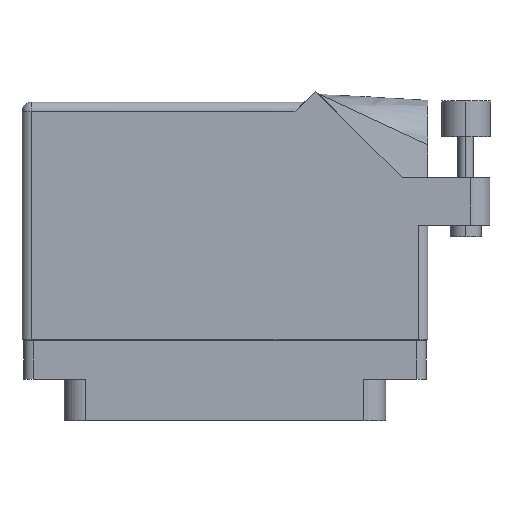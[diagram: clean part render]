
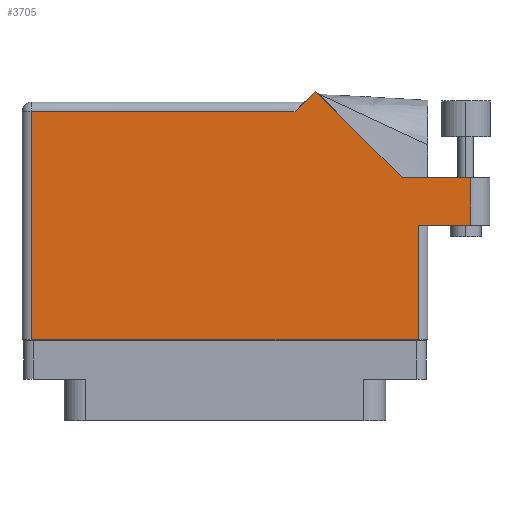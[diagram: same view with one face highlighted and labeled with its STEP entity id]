
A CAD part, front view. The second image highlights one B-rep face of the part: STEP entity #3705.
In plain terms, the highlighted face is planar.
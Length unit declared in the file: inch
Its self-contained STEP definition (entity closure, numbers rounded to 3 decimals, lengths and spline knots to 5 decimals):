
#301 = VERTEX_POINT ( 'NONE', #27446 ) ;
#938 = DIRECTION ( 'NONE',  ( 0., 1., 0. ) ) ;
#2329 = CARTESIAN_POINT ( 'NONE',  ( 1.244, 0.637, 0.455 ) ) ;
#2551 = ORIENTED_EDGE ( 'NONE', *, *, #46005, .T. ) ;
#3321 = EDGE_CURVE ( 'NONE', #7076, #5929, #33077, .T. ) ;
#3705 = ADVANCED_FACE ( 'NONE', ( #27826 ), #24356, .F. ) ;
#5131 = LINE ( 'NONE', #43101, #43248 ) ;
#5236 = VECTOR ( 'NONE', #36275, 39.37008 ) ;
#5355 = ORIENTED_EDGE ( 'NONE', *, *, #12656, .T. ) ;
#5929 = VERTEX_POINT ( 'NONE', #25314 ) ;
#6351 = CARTESIAN_POINT ( 'NONE',  ( -1.306, 1.368, 0.455 ) ) ;
#6507 = DIRECTION ( 'NONE',  ( -1., 0., 0. ) ) ;
#6863 = DIRECTION ( 'NONE',  ( 1., 0., 0. ) ) ;
#6996 = DIRECTION ( 'NONE',  ( -1., 0., 0. ) ) ;
#7076 = VERTEX_POINT ( 'NONE', #7774 ) ;
#7752 = ORIENTED_EDGE ( 'NONE', *, *, #3321, .T. ) ;
#7774 = CARTESIAN_POINT ( 'NONE',  ( 1.244, 0.637, 0.455 ) ) ;
#8053 = CARTESIAN_POINT ( 'NONE',  ( 1.581, 0.944, 0.455 ) ) ;
#8948 = ORIENTED_EDGE ( 'NONE', *, *, #35628, .T. ) ;
#9172 = LINE ( 'NONE', #17972, #5236 ) ;
#11012 = CARTESIAN_POINT ( 'NONE',  ( 1.706, 0.944, 0.455 ) ) ;
#11479 = CARTESIAN_POINT ( 'NONE',  ( -1.244, 1.368, 0.455 ) ) ;
#12656 = EDGE_CURVE ( 'NONE', #14174, #14390, #27420, .T. ) ;
#13415 = EDGE_CURVE ( 'NONE', #14390, #25380, #39496, .T. ) ;
#13550 = AXIS2_PLACEMENT_3D ( 'NONE', #39416, #39259, #17106 ) ;
#13597 = VECTOR ( 'NONE', #13934, 39.37008 ) ;
#13934 = DIRECTION ( 'NONE',  ( -0.707, -0.707, 0. ) ) ;
#14174 = VERTEX_POINT ( 'NONE', #34698 ) ;
#14390 = VERTEX_POINT ( 'NONE', #28225 ) ;
#15203 = VECTOR ( 'NONE', #6507, 39.37008 ) ;
#17106 = DIRECTION ( 'NONE',  ( -1., 0., 0. ) ) ;
#17291 = LINE ( 'NONE', #37040, #42700 ) ;
#17882 = CARTESIAN_POINT ( 'NONE',  ( 1.14042, 0.944, 0.455 ) ) ;
#17972 = CARTESIAN_POINT ( 'NONE',  ( -1.244, -0.1, 0.455 ) ) ;
#18172 = VECTOR ( 'NONE', #31569, 39.37008 ) ;
#21081 = ORIENTED_EDGE ( 'NONE', *, *, #21237, .T. ) ;
#21237 = EDGE_CURVE ( 'NONE', #5929, #301, #41864, .T. ) ;
#23212 = VECTOR ( 'NONE', #43210, 39.37008 ) ;
#24356 = PLANE ( 'NONE',  #13550 ) ;
#25314 = CARTESIAN_POINT ( 'NONE',  ( 1.581, 0.637, 0.455 ) ) ;
#25380 = VERTEX_POINT ( 'NONE', #11479 ) ;
#25832 = EDGE_CURVE ( 'NONE', #38977, #7076, #41295, .T. ) ;
#27420 = LINE ( 'NONE', #35621, #13597 ) ;
#27446 = CARTESIAN_POINT ( 'NONE',  ( 1.581, 0.944, 0.455 ) ) ;
#27452 = ORIENTED_EDGE ( 'NONE', *, *, #25832, .T. ) ;
#27723 = CARTESIAN_POINT ( 'NONE',  ( 1.306, 0.637, 0.455 ) ) ;
#27826 = FACE_OUTER_BOUND ( 'NONE', #33611, .T. ) ;
#27966 = ORIENTED_EDGE ( 'NONE', *, *, #13415, .T. ) ;
#28225 = CARTESIAN_POINT ( 'NONE',  ( 0.451, 1.368, 0.455 ) ) ;
#28959 = ORIENTED_EDGE ( 'NONE', *, *, #35350, .T. ) ;
#30722 = VERTEX_POINT ( 'NONE', #36775 ) ;
#31569 = DIRECTION ( 'NONE',  ( 0., 1., 0. ) ) ;
#33077 = LINE ( 'NONE', #27723, #23212 ) ;
#33611 = EDGE_LOOP ( 'NONE', ( #7752, #21081, #2551, #8948, #5355, #27966, #39961, #28959, #27452 ) ) ;
#34698 = CARTESIAN_POINT ( 'NONE',  ( 0.58371, 1.50071, 0.455 ) ) ;
#35350 = EDGE_CURVE ( 'NONE', #30722, #38977, #17291, .T. ) ;
#35621 = CARTESIAN_POINT ( 'NONE',  ( 0.513, 1.43, 0.455 ) ) ;
#35628 = EDGE_CURVE ( 'NONE', #43374, #14174, #5131, .T. ) ;
#36275 = DIRECTION ( 'NONE',  ( 0., -1., 0. ) ) ;
#36775 = CARTESIAN_POINT ( 'NONE',  ( -1.244, -0.1, 0.455 ) ) ;
#37040 = CARTESIAN_POINT ( 'NONE',  ( -1.306, -0.1, 0.455 ) ) ;
#37290 = VECTOR ( 'NONE', #938, 39.37008 ) ;
#37399 = LINE ( 'NONE', #11012, #40250 ) ;
#38977 = VERTEX_POINT ( 'NONE', #46409 ) ;
#39259 = DIRECTION ( 'NONE',  ( 0., 0., -1. ) ) ;
#39416 = CARTESIAN_POINT ( 'NONE',  ( -1.306, 1.43, 0.455 ) ) ;
#39496 = LINE ( 'NONE', #6351, #15203 ) ;
#39961 = ORIENTED_EDGE ( 'NONE', *, *, #43880, .T. ) ;
#40250 = VECTOR ( 'NONE', #6996, 39.37008 ) ;
#41123 = DIRECTION ( 'NONE',  ( -0.707, 0.707, 0. ) ) ;
#41295 = LINE ( 'NONE', #2329, #18172 ) ;
#41864 = LINE ( 'NONE', #8053, #37290 ) ;
#42700 = VECTOR ( 'NONE', #6863, 39.37008 ) ;
#43101 = CARTESIAN_POINT ( 'NONE',  ( 1.14042, 0.944, 0.455 ) ) ;
#43210 = DIRECTION ( 'NONE',  ( 1., 0., 0. ) ) ;
#43248 = VECTOR ( 'NONE', #41123, 39.37008 ) ;
#43374 = VERTEX_POINT ( 'NONE', #17882 ) ;
#43880 = EDGE_CURVE ( 'NONE', #25380, #30722, #9172, .T. ) ;
#46005 = EDGE_CURVE ( 'NONE', #301, #43374, #37399, .T. ) ;
#46409 = CARTESIAN_POINT ( 'NONE',  ( 1.244, -0.1, 0.455 ) ) ;
